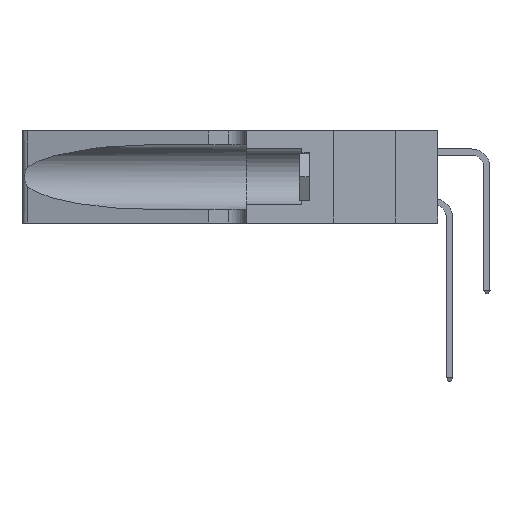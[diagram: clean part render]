
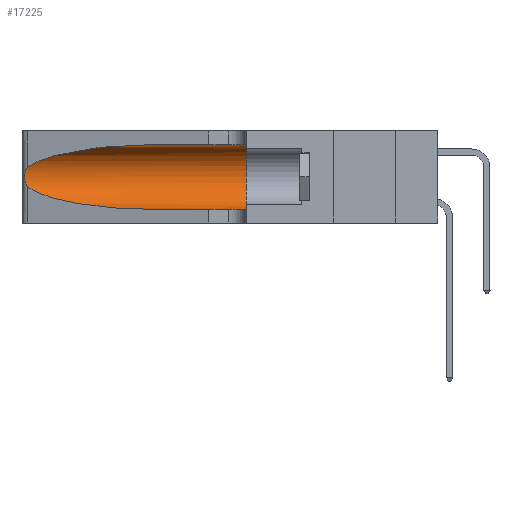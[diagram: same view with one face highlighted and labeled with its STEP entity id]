
A CAD part, left-side view. The second image highlights one B-rep face of the part: STEP entity #17225.
In plain terms, the highlighted cylindrical face has radius 3.308 mm (diameter 6.617 mm), a partial arc.
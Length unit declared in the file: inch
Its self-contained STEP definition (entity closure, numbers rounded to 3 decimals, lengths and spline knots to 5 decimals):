
#1244 = CARTESIAN_POINT ( 'NONE',  ( 0.25487, 1.22718, 0.22369 ) ) ;
#1411 = CARTESIAN_POINT ( 'NONE',  ( 0.25854, 1.2359, 0.20912 ) ) ;
#1739 = CARTESIAN_POINT ( 'NONE',  ( 0.25555, 1.22994, 0.2215 ) ) ;
#2905 = CARTESIAN_POINT ( 'NONE',  ( 0.25487, 1.22718, 0.22369 ) ) ;
#4411 = CARTESIAN_POINT ( 'NONE',  ( 0.25487, 1.22718, 0.14631 ) ) ;
#5162 = LINE ( 'NONE', #15738, #21641 ) ;
#5177 = CARTESIAN_POINT ( 'NONE',  ( 0.1305, 1.61858, 0.31525 ) ) ;
#5547 = CARTESIAN_POINT ( 'NONE',  ( 0.26075, 1.23896, 0.19203 ) ) ;
#7214 = B_SPLINE_CURVE_WITH_KNOTS ( 'NONE', 3,
 ( #16374, #1739, #11235, #30739, #1411, #24307, #5547, #18165, #26292, #16445, #16655, #9110, #24538, #8250 ),
 .UNSPECIFIED., .F., .F.,
 ( 4, 2, 2, 2, 2, 2, 4 ),
 ( 0., 0.00027, 0.00053, 0.00107, 0.0016, 0.00187, 0.00214 ),
 .UNSPECIFIED. ) ;
#7503 = CARTESIAN_POINT ( 'NONE',  ( 0.25487, 1.22718, 0.14631 ) ) ;
#7923 = DIRECTION ( 'NONE',  ( 0., 1., 0. ) ) ;
#8250 = CARTESIAN_POINT ( 'NONE',  ( 0.25487, 1.22718, 0.14631 ) ) ;
#9110 = CARTESIAN_POINT ( 'NONE',  ( 0.25639, 1.23186, 0.15144 ) ) ;
#9113 = DIRECTION ( 'NONE',  ( 0., -1., 0. ) ) ;
#10046 = DIRECTION ( 'NONE',  ( 0., 0., -1. ) ) ;
#11235 = CARTESIAN_POINT ( 'NONE',  ( 0.25639, 1.23184, 0.21858 ) ) ;
#11320 = VERTEX_POINT ( 'NONE', #13369 ) ;
#11392 = EDGE_CURVE ( 'NONE', #20105, #18412, #7214, .T. ) ;
#11951 = EDGE_CURVE ( 'NONE', #17238, #15004, #15941, .T. ) ;
#12405 = CARTESIAN_POINT ( 'NONE',  ( 0.2373, 1.15595, 0.28018 ) ) ;
#13369 = CARTESIAN_POINT ( 'NONE',  ( 0.1305, 0.72297, 0.31525 ) ) ;
#13488 = AXIS2_PLACEMENT_3D ( 'NONE', #13881, #19808, #10046 ) ;
#13881 = CARTESIAN_POINT ( 'NONE',  ( 0.1305, 1.61858, 0.185 ) ) ;
#14875 = CARTESIAN_POINT ( 'NONE',  ( 0.1305, 0.72297, 0.05475 ) ) ;
#15004 = VERTEX_POINT ( 'NONE', #29083 ) ;
#15401 = CARTESIAN_POINT ( 'NONE',  ( 0.1305, 0.35, 0.185 ) ) ;
#15738 = CARTESIAN_POINT ( 'NONE',  ( 0.1305, 1.61858, 0.05475 ) ) ;
#15941 = CIRCLE ( 'NONE', #28966, 0.13025 ) ;
#16131 = ORIENTED_EDGE ( 'NONE', *, *, #11951, .F. ) ;
#16317 = ORIENTED_EDGE ( 'NONE', *, *, #11392, .T. ) ;
#16374 = CARTESIAN_POINT ( 'NONE',  ( 0.25487, 1.22718, 0.22369 ) ) ;
#16445 = CARTESIAN_POINT ( 'NONE',  ( 0.25856, 1.23593, 0.16098 ) ) ;
#16655 = CARTESIAN_POINT ( 'NONE',  ( 0.25789, 1.23486, 0.15765 ) ) ;
#17225 = ADVANCED_FACE ( 'NONE', ( #22956 ), #31025, .F. ) ;
#17238 = VERTEX_POINT ( 'NONE', #21515 ) ;
#17326 = ORIENTED_EDGE ( 'NONE', *, *, #18633, .T. ) ;
#17444 = CARTESIAN_POINT ( 'NONE',  ( 0.18966, 0.96281, 0.05475 ) ) ;
#17543 = CARTESIAN_POINT ( 'NONE',  ( 0.18966, 0.96281, 0.31525 ) ) ;
#18024 = ORIENTED_EDGE ( 'NONE', *, *, #22674, .T. ) ;
#18165 = CARTESIAN_POINT ( 'NONE',  ( 0.26075, 1.23896, 0.178 ) ) ;
#18412 = VERTEX_POINT ( 'NONE', #4411 ) ;
#18633 = EDGE_CURVE ( 'NONE', #11320, #20105, #20021, .T. ) ;
#18637 = EDGE_CURVE ( 'NONE', #18412, #21725, #28053, .T. ) ;
#19737 = CARTESIAN_POINT ( 'NONE',  ( 0.1305, 0.72297, 0.31525 ) ) ;
#19808 = DIRECTION ( 'NONE',  ( 0., -1., 0. ) ) ;
#19986 = DIRECTION ( 'NONE',  ( 0., -1., 0. ) ) ;
#20021 =( BOUNDED_CURVE ( )  B_SPLINE_CURVE ( 3, ( #19737, #17543, #12405, #2905 ),
 .UNSPECIFIED., .F., .F. ) 
 B_SPLINE_CURVE_WITH_KNOTS ( ( 4, 4 ),
 ( 1.5708, 2.84003 ),
 .UNSPECIFIED. ) 
 CURVE ( )  GEOMETRIC_REPRESENTATION_ITEM ( )  RATIONAL_B_SPLINE_CURVE ( ( 1., 0.87, 0.87, 1. ) ) 
 REPRESENTATION_ITEM ( '' )  );
#20105 = VERTEX_POINT ( 'NONE', #1244 ) ;
#20348 = EDGE_CURVE ( 'NONE', #11320, #17238, #30478, .T. ) ;
#20468 = ORIENTED_EDGE ( 'NONE', *, *, #20348, .F. ) ;
#21515 = CARTESIAN_POINT ( 'NONE',  ( 0.1305, 0.35, 0.31525 ) ) ;
#21641 = VECTOR ( 'NONE', #9113, 39.37008 ) ;
#21725 = VERTEX_POINT ( 'NONE', #27382 ) ;
#22674 = EDGE_CURVE ( 'NONE', #21725, #15004, #5162, .T. ) ;
#22956 = FACE_OUTER_BOUND ( 'NONE', #31708, .T. ) ;
#23465 = DIRECTION ( 'NONE',  ( 0., 0., 1. ) ) ;
#24307 = CARTESIAN_POINT ( 'NONE',  ( 0.26018, 1.23835, 0.19895 ) ) ;
#24432 = ORIENTED_EDGE ( 'NONE', *, *, #18637, .T. ) ;
#24538 = CARTESIAN_POINT ( 'NONE',  ( 0.25555, 1.22993, 0.14849 ) ) ;
#24736 = VECTOR ( 'NONE', #19986, 39.37008 ) ;
#26292 = CARTESIAN_POINT ( 'NONE',  ( 0.26017, 1.23833, 0.17102 ) ) ;
#27382 = CARTESIAN_POINT ( 'NONE',  ( 0.1305, 0.72297, 0.05475 ) ) ;
#28053 =( BOUNDED_CURVE ( )  B_SPLINE_CURVE ( 3, ( #7503, #29573, #17444, #14875 ),
 .UNSPECIFIED., .F., .T. ) 
 B_SPLINE_CURVE_WITH_KNOTS ( ( 4, 4 ),
 ( 3.44316, 4.71239 ),
 .UNSPECIFIED. ) 
 CURVE ( )  GEOMETRIC_REPRESENTATION_ITEM ( )  RATIONAL_B_SPLINE_CURVE ( ( 1., 0.87, 0.87, 1. ) ) 
 REPRESENTATION_ITEM ( '' )  );
#28966 = AXIS2_PLACEMENT_3D ( 'NONE', #15401, #7923, #23465 ) ;
#29083 = CARTESIAN_POINT ( 'NONE',  ( 0.1305, 0.35, 0.05475 ) ) ;
#29573 = CARTESIAN_POINT ( 'NONE',  ( 0.2373, 1.15595, 0.08982 ) ) ;
#30478 = LINE ( 'NONE', #5177, #24736 ) ;
#30739 = CARTESIAN_POINT ( 'NONE',  ( 0.25787, 1.23484, 0.2124 ) ) ;
#31025 = CYLINDRICAL_SURFACE ( 'NONE', #13488, 0.13025 ) ;
#31708 = EDGE_LOOP ( 'NONE', ( #17326, #16317, #24432, #18024, #16131, #20468 ) ) ;
